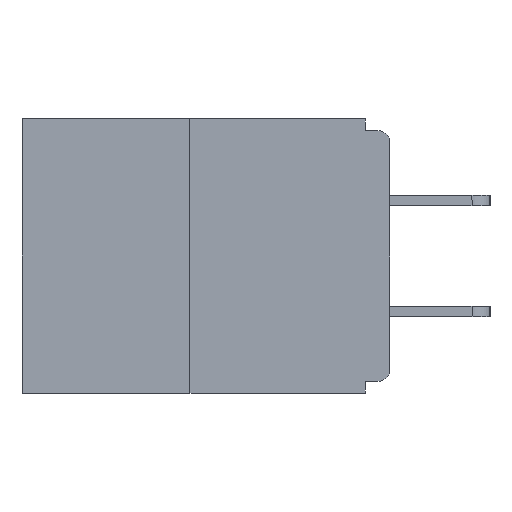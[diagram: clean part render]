
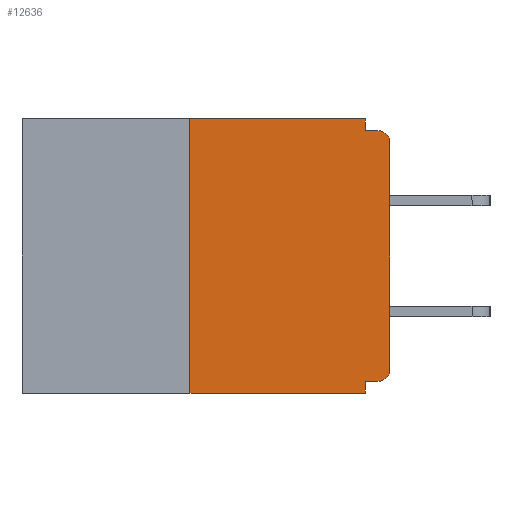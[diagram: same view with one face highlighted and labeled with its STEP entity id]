
A CAD part, left-side view. The second image highlights one B-rep face of the part: STEP entity #12636.
In plain terms, the highlighted planar face has unit normal (-1, 0, 0).
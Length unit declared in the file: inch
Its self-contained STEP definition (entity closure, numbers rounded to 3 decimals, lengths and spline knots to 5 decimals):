
#252 = AXIS2_PLACEMENT_3D ( 'NONE', #21245, #23993, #1685 ) ;
#454 = EDGE_CURVE ( 'NONE', #25542, #11881, #19818, .T. ) ;
#471 = VERTEX_POINT ( 'NONE', #8758 ) ;
#806 = VERTEX_POINT ( 'NONE', #19140 ) ;
#851 = CARTESIAN_POINT ( 'NONE',  ( 0., 0.031, 0. ) ) ;
#888 = DIRECTION ( 'NONE',  ( 0., -1., 0. ) ) ;
#1048 = LINE ( 'NONE', #9857, #15545 ) ;
#1357 = FACE_OUTER_BOUND ( 'NONE', #25420, .T. ) ;
#1685 = DIRECTION ( 'NONE',  ( 0., 0., -1. ) ) ;
#1692 = CARTESIAN_POINT ( 'NONE',  ( 0., 0.46, 0. ) ) ;
#2479 = ORIENTED_EDGE ( 'NONE', *, *, #454, .F. ) ;
#3287 = CARTESIAN_POINT ( 'NONE',  ( 0., 0., -0.03 ) ) ;
#3401 = DIRECTION ( 'NONE',  ( -1., 0., 0. ) ) ;
#3402 = CARTESIAN_POINT ( 'NONE',  ( 0., 0., -0.015 ) ) ;
#3487 = DIRECTION ( 'NONE',  ( 0., 0., -1. ) ) ;
#4106 = ORIENTED_EDGE ( 'NONE', *, *, #13965, .T. ) ;
#4267 = EDGE_CURVE ( 'NONE', #471, #24651, #1048, .T. ) ;
#4430 = DIRECTION ( 'NONE',  ( 0., 0., -1. ) ) ;
#4618 = VECTOR ( 'NONE', #4430, 39.37008 ) ;
#4684 = AXIS2_PLACEMENT_3D ( 'NONE', #5552, #3401, #3487 ) ;
#5552 = CARTESIAN_POINT ( 'NONE',  ( 0., 0.015, -0.03 ) ) ;
#6265 = ORIENTED_EDGE ( 'NONE', *, *, #23092, .T. ) ;
#6684 = VERTEX_POINT ( 'NONE', #3287 ) ;
#7016 = CIRCLE ( 'NONE', #252, 0.015 ) ;
#7161 = VECTOR ( 'NONE', #27982, 39.37008 ) ;
#7426 = VERTEX_POINT ( 'NONE', #19667 ) ;
#7681 = CARTESIAN_POINT ( 'NONE',  ( 0., 0., 0. ) ) ;
#8465 = CARTESIAN_POINT ( 'NONE',  ( 0., 0.031, -0.343 ) ) ;
#8679 = VERTEX_POINT ( 'NONE', #25072 ) ;
#8682 = EDGE_CURVE ( 'NONE', #6684, #8679, #22551, .T. ) ;
#8758 = CARTESIAN_POINT ( 'NONE',  ( 0., 0.25, 0. ) ) ;
#9373 = ORIENTED_EDGE ( 'NONE', *, *, #8682, .T. ) ;
#9581 = DIRECTION ( 'NONE',  ( 0., -1., 0. ) ) ;
#9857 = CARTESIAN_POINT ( 'NONE',  ( 0., 0.46, 0. ) ) ;
#10099 = CARTESIAN_POINT ( 'NONE',  ( 0., 0.031, -0.328 ) ) ;
#10251 = DIRECTION ( 'NONE',  ( 0., 0., 1. ) ) ;
#10378 = DIRECTION ( 'NONE',  ( 0., 0., -1. ) ) ;
#11099 = LINE ( 'NONE', #26666, #26338 ) ;
#11412 = ORIENTED_EDGE ( 'NONE', *, *, #21449, .F. ) ;
#11543 = LINE ( 'NONE', #16061, #22050 ) ;
#11881 = VERTEX_POINT ( 'NONE', #8465 ) ;
#11962 = LINE ( 'NONE', #13159, #17029 ) ;
#12636 = ADVANCED_FACE ( 'NONE', ( #1357 ), #14511, .F. ) ;
#13159 = CARTESIAN_POINT ( 'NONE',  ( 0., 0.25, 0. ) ) ;
#13833 = VERTEX_POINT ( 'NONE', #15638 ) ;
#13965 = EDGE_CURVE ( 'NONE', #13833, #20224, #7016, .T. ) ;
#14283 = VECTOR ( 'NONE', #20774, 39.37008 ) ;
#14511 = PLANE ( 'NONE',  #16489 ) ;
#14683 = CARTESIAN_POINT ( 'NONE',  ( 0., 0.031, 0. ) ) ;
#14992 = CARTESIAN_POINT ( 'NONE',  ( 0., 0.031, -0.343 ) ) ;
#15545 = VECTOR ( 'NONE', #9581, 39.37008 ) ;
#15638 = CARTESIAN_POINT ( 'NONE',  ( 0., 0.015, -0.328 ) ) ;
#15798 = CARTESIAN_POINT ( 'NONE',  ( 0., 0., -0.313 ) ) ;
#16061 = CARTESIAN_POINT ( 'NONE',  ( 0., 0.46, -0.343 ) ) ;
#16489 = AXIS2_PLACEMENT_3D ( 'NONE', #1692, #25520, #10378 ) ;
#17029 = VECTOR ( 'NONE', #26397, 39.37008 ) ;
#19045 = ORIENTED_EDGE ( 'NONE', *, *, #22481, .T. ) ;
#19140 = CARTESIAN_POINT ( 'NONE',  ( 0., 0.25, -0.343 ) ) ;
#19307 = LINE ( 'NONE', #7681, #23389 ) ;
#19667 = CARTESIAN_POINT ( 'NONE',  ( 0., 0.031, -0.015 ) ) ;
#19787 = ORIENTED_EDGE ( 'NONE', *, *, #22225, .F. ) ;
#19818 = LINE ( 'NONE', #14992, #4618 ) ;
#20224 = VERTEX_POINT ( 'NONE', #15798 ) ;
#20774 = DIRECTION ( 'NONE',  ( 0., -1., 0. ) ) ;
#21245 = CARTESIAN_POINT ( 'NONE',  ( 0., 0.015, -0.313 ) ) ;
#21449 = EDGE_CURVE ( 'NONE', #806, #471, #11962, .T. ) ;
#21695 = EDGE_CURVE ( 'NONE', #7426, #8679, #26499, .T. ) ;
#22050 = VECTOR ( 'NONE', #888, 39.37008 ) ;
#22225 = EDGE_CURVE ( 'NONE', #24651, #7426, #23764, .T. ) ;
#22388 = DIRECTION ( 'NONE',  ( 0., 1., 0. ) ) ;
#22481 = EDGE_CURVE ( 'NONE', #806, #11881, #11543, .T. ) ;
#22551 = CIRCLE ( 'NONE', #4684, 0.015 ) ;
#23092 = EDGE_CURVE ( 'NONE', #20224, #6684, #19307, .T. ) ;
#23389 = VECTOR ( 'NONE', #10251, 39.37008 ) ;
#23764 = LINE ( 'NONE', #14683, #7161 ) ;
#23993 = DIRECTION ( 'NONE',  ( -1., 0., 0. ) ) ;
#24032 = ORIENTED_EDGE ( 'NONE', *, *, #27381, .F. ) ;
#24651 = VERTEX_POINT ( 'NONE', #851 ) ;
#25072 = CARTESIAN_POINT ( 'NONE',  ( 0., 0.015, -0.015 ) ) ;
#25420 = EDGE_LOOP ( 'NONE', ( #27768, #11412, #19045, #2479, #24032, #4106, #6265, #9373, #27533, #19787 ) ) ;
#25520 = DIRECTION ( 'NONE',  ( 1., 0., 0. ) ) ;
#25542 = VERTEX_POINT ( 'NONE', #10099 ) ;
#26338 = VECTOR ( 'NONE', #22388, 39.37008 ) ;
#26397 = DIRECTION ( 'NONE',  ( 0., 0., 1. ) ) ;
#26499 = LINE ( 'NONE', #3402, #14283 ) ;
#26666 = CARTESIAN_POINT ( 'NONE',  ( 0., 0., -0.328 ) ) ;
#27381 = EDGE_CURVE ( 'NONE', #13833, #25542, #11099, .T. ) ;
#27533 = ORIENTED_EDGE ( 'NONE', *, *, #21695, .F. ) ;
#27768 = ORIENTED_EDGE ( 'NONE', *, *, #4267, .F. ) ;
#27982 = DIRECTION ( 'NONE',  ( 0., 0., -1. ) ) ;
